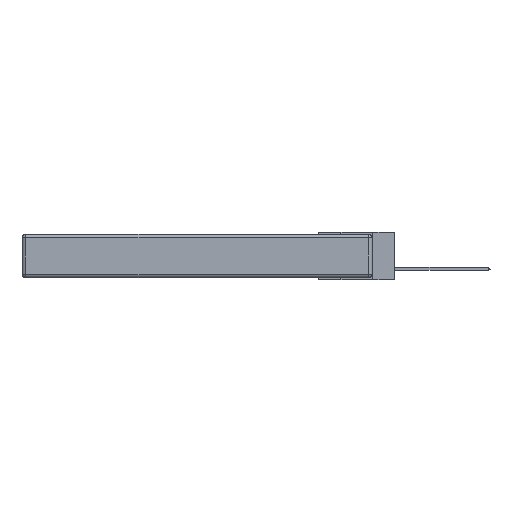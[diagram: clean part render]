
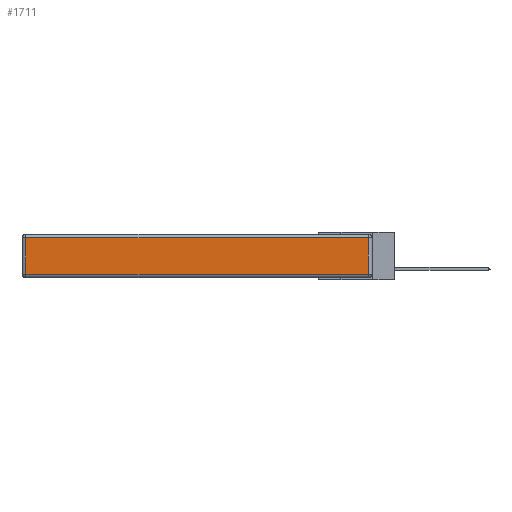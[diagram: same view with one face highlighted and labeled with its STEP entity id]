
A CAD part, left-side view. The second image highlights one B-rep face of the part: STEP entity #1711.
In plain terms, the highlighted planar face has unit normal (-1, 0, 0).
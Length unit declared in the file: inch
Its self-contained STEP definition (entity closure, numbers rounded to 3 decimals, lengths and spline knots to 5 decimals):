
#403 = DIRECTION ( 'NONE',  ( 0., -1., 0. ) ) ;
#1014 = ORIENTED_EDGE ( 'NONE', *, *, #20277, .T. ) ;
#1623 = VERTEX_POINT ( 'NONE', #4331 ) ;
#1711 = ADVANCED_FACE ( 'NONE', ( #5672 ), #19115, .T. ) ;
#2024 = DIRECTION ( 'NONE',  ( -1., 0., 0. ) ) ;
#4331 = CARTESIAN_POINT ( 'NONE',  ( 0., 2.72, -0.03 ) ) ;
#4426 = VECTOR ( 'NONE', #4739, 39.37008 ) ;
#4739 = DIRECTION ( 'NONE',  ( 0., 0., -1. ) ) ;
#5152 = VECTOR ( 'NONE', #11659, 39.37008 ) ;
#5485 = LINE ( 'NONE', #8542, #20032 ) ;
#5672 = FACE_OUTER_BOUND ( 'NONE', #19072, .T. ) ;
#6552 = CARTESIAN_POINT ( 'NONE',  ( 0., 2.75, -0.03 ) ) ;
#7076 = LINE ( 'NONE', #11564, #4426 ) ;
#7446 = ORIENTED_EDGE ( 'NONE', *, *, #14478, .T. ) ;
#8542 = CARTESIAN_POINT ( 'NONE',  ( 0., 0., -0.313 ) ) ;
#8544 = ORIENTED_EDGE ( 'NONE', *, *, #18009, .T. ) ;
#8759 = AXIS2_PLACEMENT_3D ( 'NONE', #17366, #2024, #10539 ) ;
#9810 = DIRECTION ( 'NONE',  ( 0., 0., 1. ) ) ;
#9823 = VERTEX_POINT ( 'NONE', #13151 ) ;
#10539 = DIRECTION ( 'NONE',  ( 0., 0., 1. ) ) ;
#10574 = VERTEX_POINT ( 'NONE', #20431 ) ;
#11527 = LINE ( 'NONE', #6552, #5152 ) ;
#11564 = CARTESIAN_POINT ( 'NONE',  ( 0., 2.72, -0.343 ) ) ;
#11659 = DIRECTION ( 'NONE',  ( 0., 1., 0. ) ) ;
#12159 = VECTOR ( 'NONE', #9810, 39.37008 ) ;
#12992 = CARTESIAN_POINT ( 'NONE',  ( 0., 0.03, -0.343 ) ) ;
#13151 = CARTESIAN_POINT ( 'NONE',  ( 0., 2.72, -0.313 ) ) ;
#14478 = EDGE_CURVE ( 'NONE', #10574, #1623, #11527, .T. ) ;
#16298 = VERTEX_POINT ( 'NONE', #20145 ) ;
#16394 = ORIENTED_EDGE ( 'NONE', *, *, #20686, .T. ) ;
#17366 = CARTESIAN_POINT ( 'NONE',  ( 0., 0., -0.343 ) ) ;
#18009 = EDGE_CURVE ( 'NONE', #16298, #10574, #21645, .T. ) ;
#19072 = EDGE_LOOP ( 'NONE', ( #1014, #8544, #7446, #16394 ) ) ;
#19115 = PLANE ( 'NONE',  #8759 ) ;
#20032 = VECTOR ( 'NONE', #403, 39.37008 ) ;
#20145 = CARTESIAN_POINT ( 'NONE',  ( 0., 0.03, -0.313 ) ) ;
#20277 = EDGE_CURVE ( 'NONE', #9823, #16298, #5485, .T. ) ;
#20431 = CARTESIAN_POINT ( 'NONE',  ( 0., 0.03, -0.03 ) ) ;
#20686 = EDGE_CURVE ( 'NONE', #1623, #9823, #7076, .T. ) ;
#21645 = LINE ( 'NONE', #12992, #12159 ) ;
